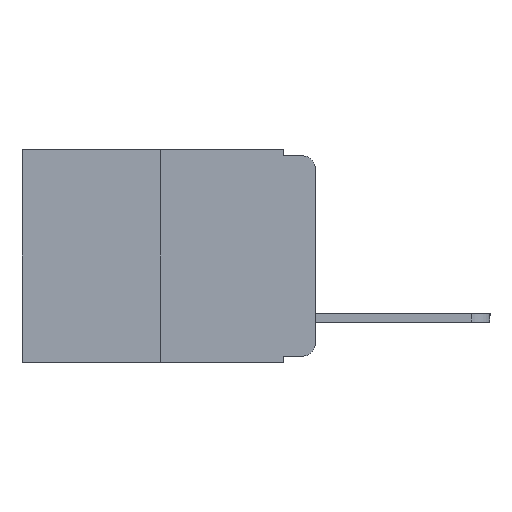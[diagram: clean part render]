
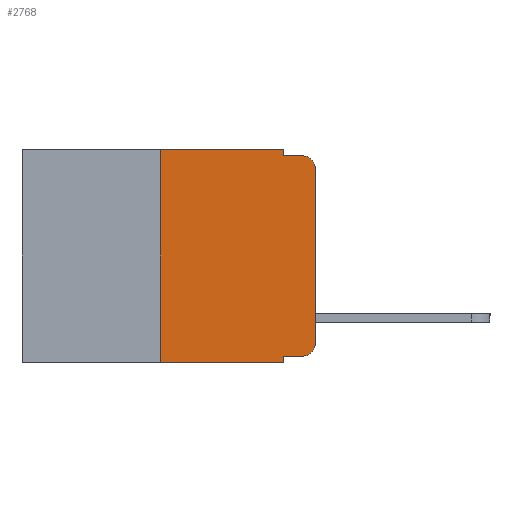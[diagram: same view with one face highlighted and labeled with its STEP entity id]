
A CAD part, left-side view. The second image highlights one B-rep face of the part: STEP entity #2768.
In plain terms, the highlighted planar face has unit normal (-1, 0, 0).
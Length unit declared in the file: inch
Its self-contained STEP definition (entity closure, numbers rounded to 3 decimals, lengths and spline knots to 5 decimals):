
#7 = ORIENTED_EDGE ( 'NONE', *, *, #3635, .F. ) ;
#109 = LINE ( 'NONE', #12739, #6321 ) ;
#243 = LINE ( 'NONE', #3021, #9595 ) ;
#638 = VERTEX_POINT ( 'NONE', #12362 ) ;
#849 = CARTESIAN_POINT ( 'NONE',  ( 0., 0., -0.03 ) ) ;
#977 = CARTESIAN_POINT ( 'NONE',  ( 0., 0.25, -0.343 ) ) ;
#1361 = VECTOR ( 'NONE', #6353, 39.37008 ) ;
#1473 = CARTESIAN_POINT ( 'NONE',  ( 0., 0.051, 0. ) ) ;
#1531 = CARTESIAN_POINT ( 'NONE',  ( 0., 0.02, -0.03 ) ) ;
#1661 = VERTEX_POINT ( 'NONE', #5863 ) ;
#1765 = VECTOR ( 'NONE', #12246, 39.37008 ) ;
#1893 = VERTEX_POINT ( 'NONE', #977 ) ;
#2280 = AXIS2_PLACEMENT_3D ( 'NONE', #11347, #10836, #10823 ) ;
#2324 = VECTOR ( 'NONE', #5268, 39.37008 ) ;
#2768 = ADVANCED_FACE ( 'NONE', ( #5045 ), #11263, .F. ) ;
#2783 = DIRECTION ( 'NONE',  ( 0., 0., -1. ) ) ;
#3012 = ORIENTED_EDGE ( 'NONE', *, *, #6053, .T. ) ;
#3021 = CARTESIAN_POINT ( 'NONE',  ( 0., 0.051, -0.333 ) ) ;
#3623 = VERTEX_POINT ( 'NONE', #4504 ) ;
#3635 = EDGE_CURVE ( 'NONE', #3623, #9545, #4071, .T. ) ;
#4071 = LINE ( 'NONE', #7020, #9355 ) ;
#4306 = CARTESIAN_POINT ( 'NONE',  ( 0., 0.473, -0.343 ) ) ;
#4440 = EDGE_CURVE ( 'NONE', #12948, #1661, #5533, .T. ) ;
#4504 = CARTESIAN_POINT ( 'NONE',  ( 0., 0.25, 0. ) ) ;
#4639 = LINE ( 'NONE', #9522, #1361 ) ;
#4713 = CARTESIAN_POINT ( 'NONE',  ( 0., 0.02, -0.333 ) ) ;
#5045 = FACE_OUTER_BOUND ( 'NONE', #6344, .T. ) ;
#5209 = EDGE_CURVE ( 'NONE', #8952, #12978, #12043, .T. ) ;
#5229 = EDGE_CURVE ( 'NONE', #12948, #8952, #243, .T. ) ;
#5268 = DIRECTION ( 'NONE',  ( 0., 0., -1. ) ) ;
#5533 = LINE ( 'NONE', #8625, #2324 ) ;
#5826 = EDGE_CURVE ( 'NONE', #1893, #3623, #109, .T. ) ;
#5863 = CARTESIAN_POINT ( 'NONE',  ( 0., 0.051, -0.343 ) ) ;
#6046 = EDGE_CURVE ( 'NONE', #9545, #11882, #13023, .T. ) ;
#6050 = EDGE_CURVE ( 'NONE', #11882, #638, #4639, .T. ) ;
#6053 = EDGE_CURVE ( 'NONE', #13746, #638, #7738, .T. ) ;
#6095 = EDGE_CURVE ( 'NONE', #12978, #13746, #7021, .T. ) ;
#6228 = ORIENTED_EDGE ( 'NONE', *, *, #6046, .F. ) ;
#6321 = VECTOR ( 'NONE', #11855, 39.37008 ) ;
#6344 = EDGE_LOOP ( 'NONE', ( #8801, #3012, #9113, #6228, #7, #6936, #6573, #10010, #7652, #12408 ) ) ;
#6353 = DIRECTION ( 'NONE',  ( 0., -1., 0. ) ) ;
#6573 = ORIENTED_EDGE ( 'NONE', *, *, #11409, .T. ) ;
#6578 = DIRECTION ( 'NONE',  ( -1., 0., 0. ) ) ;
#6608 = CARTESIAN_POINT ( 'NONE',  ( 0., 0.051, -0.333 ) ) ;
#6936 = ORIENTED_EDGE ( 'NONE', *, *, #5826, .F. ) ;
#7020 = CARTESIAN_POINT ( 'NONE',  ( 0., 0.473, 0. ) ) ;
#7021 = LINE ( 'NONE', #7649, #10081 ) ;
#7174 = CARTESIAN_POINT ( 'NONE',  ( 0., 0.051, -0.01 ) ) ;
#7610 = VECTOR ( 'NONE', #7828, 39.37008 ) ;
#7649 = CARTESIAN_POINT ( 'NONE',  ( 0., 0., 0. ) ) ;
#7652 = ORIENTED_EDGE ( 'NONE', *, *, #5229, .T. ) ;
#7732 = DIRECTION ( 'NONE',  ( 0., -1., 0. ) ) ;
#7738 = CIRCLE ( 'NONE', #13191, 0.02 ) ;
#7828 = DIRECTION ( 'NONE',  ( 0., -1., 0. ) ) ;
#8009 = CARTESIAN_POINT ( 'NONE',  ( 0., 0.051, 0. ) ) ;
#8310 = LINE ( 'NONE', #4306, #7610 ) ;
#8625 = CARTESIAN_POINT ( 'NONE',  ( 0., 0.051, 0. ) ) ;
#8801 = ORIENTED_EDGE ( 'NONE', *, *, #6095, .T. ) ;
#8952 = VERTEX_POINT ( 'NONE', #4713 ) ;
#9113 = ORIENTED_EDGE ( 'NONE', *, *, #6050, .F. ) ;
#9355 = VECTOR ( 'NONE', #12592, 39.37008 ) ;
#9522 = CARTESIAN_POINT ( 'NONE',  ( 0., 0.051, -0.01 ) ) ;
#9545 = VERTEX_POINT ( 'NONE', #8009 ) ;
#9565 = DIRECTION ( 'NONE',  ( -1., 0., 0. ) ) ;
#9595 = VECTOR ( 'NONE', #7732, 39.37008 ) ;
#10010 = ORIENTED_EDGE ( 'NONE', *, *, #4440, .F. ) ;
#10081 = VECTOR ( 'NONE', #10575, 39.37008 ) ;
#10575 = DIRECTION ( 'NONE',  ( 0., 0., 1. ) ) ;
#10823 = DIRECTION ( 'NONE',  ( 0., 0., -1. ) ) ;
#10836 = DIRECTION ( 'NONE',  ( 1., 0., 0. ) ) ;
#11263 = PLANE ( 'NONE',  #2280 ) ;
#11347 = CARTESIAN_POINT ( 'NONE',  ( 0., 0.473, 0. ) ) ;
#11409 = EDGE_CURVE ( 'NONE', #1893, #1661, #8310, .T. ) ;
#11623 = CARTESIAN_POINT ( 'NONE',  ( 0., 0., -0.313 ) ) ;
#11855 = DIRECTION ( 'NONE',  ( 0., 0., 1. ) ) ;
#11882 = VERTEX_POINT ( 'NONE', #7174 ) ;
#12043 = CIRCLE ( 'NONE', #13463, 0.02 ) ;
#12246 = DIRECTION ( 'NONE',  ( 0., 0., -1. ) ) ;
#12362 = CARTESIAN_POINT ( 'NONE',  ( 0., 0.02, -0.01 ) ) ;
#12408 = ORIENTED_EDGE ( 'NONE', *, *, #5209, .T. ) ;
#12452 = CARTESIAN_POINT ( 'NONE',  ( 0., 0.02, -0.313 ) ) ;
#12592 = DIRECTION ( 'NONE',  ( 0., -1., 0. ) ) ;
#12739 = CARTESIAN_POINT ( 'NONE',  ( 0., 0.25, 0. ) ) ;
#12948 = VERTEX_POINT ( 'NONE', #6608 ) ;
#12978 = VERTEX_POINT ( 'NONE', #11623 ) ;
#13023 = LINE ( 'NONE', #1473, #1765 ) ;
#13191 = AXIS2_PLACEMENT_3D ( 'NONE', #1531, #9565, #2783 ) ;
#13294 = DIRECTION ( 'NONE',  ( 0., 0., -1. ) ) ;
#13463 = AXIS2_PLACEMENT_3D ( 'NONE', #12452, #6578, #13294 ) ;
#13746 = VERTEX_POINT ( 'NONE', #849 ) ;
